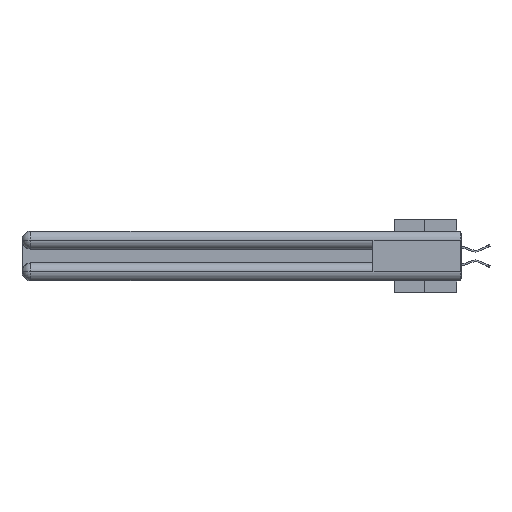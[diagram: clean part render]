
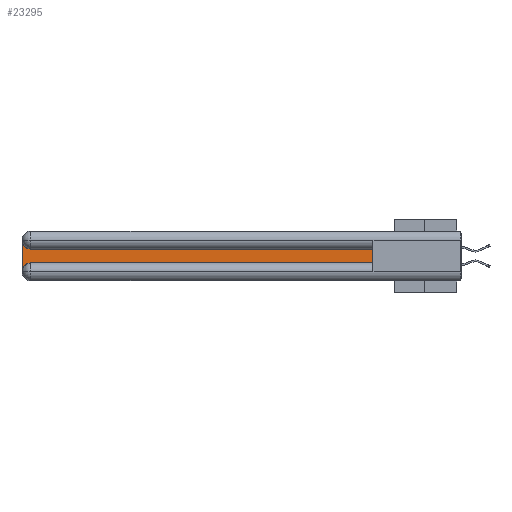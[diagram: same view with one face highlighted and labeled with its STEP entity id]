
A CAD part, left-side view. The second image highlights one B-rep face of the part: STEP entity #23295.
In plain terms, the highlighted planar face has unit normal (-1, 0, 0).
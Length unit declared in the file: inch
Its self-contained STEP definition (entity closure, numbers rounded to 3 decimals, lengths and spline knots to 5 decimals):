
#2069 = ORIENTED_EDGE ( 'NONE', *, *, #46272, .T. ) ;
#2218 = CIRCLE ( 'NONE', #29656, 0.06 ) ;
#2389 = CARTESIAN_POINT ( 'NONE',  ( 0.075, 0.6, -0.1225 ) ) ;
#2857 = LINE ( 'NONE', #18264, #46001 ) ;
#3168 = ORIENTED_EDGE ( 'NONE', *, *, #39112, .T. ) ;
#5815 = DIRECTION ( 'NONE',  ( 0., 1., 0. ) ) ;
#6115 = VERTEX_POINT ( 'NONE', #44631 ) ;
#7682 = DIRECTION ( 'NONE',  ( 1., 0., 0. ) ) ;
#7932 = CARTESIAN_POINT ( 'NONE',  ( 0.075, 2.94, -0.0625 ) ) ;
#8940 = VERTEX_POINT ( 'NONE', #38686 ) ;
#10243 = CARTESIAN_POINT ( 'NONE',  ( 0.075, 3., -0.2175 ) ) ;
#10977 = CARTESIAN_POINT ( 'NONE',  ( 0.075, 3., -0.2775 ) ) ;
#11154 = VERTEX_POINT ( 'NONE', #20081 ) ;
#11517 = DIRECTION ( 'NONE',  ( 0., 0., -1. ) ) ;
#12736 = FACE_OUTER_BOUND ( 'NONE', #31958, .T. ) ;
#13480 = ORIENTED_EDGE ( 'NONE', *, *, #30019, .T. ) ;
#13615 = AXIS2_PLACEMENT_3D ( 'NONE', #16270, #34154, #30084 ) ;
#15147 = DIRECTION ( 'NONE',  ( 0., 0., -1. ) ) ;
#15206 = ORIENTED_EDGE ( 'NONE', *, *, #25085, .T. ) ;
#16270 = CARTESIAN_POINT ( 'NONE',  ( 0.075, 3., -0.1225 ) ) ;
#16906 = VERTEX_POINT ( 'NONE', #38642 ) ;
#18264 = CARTESIAN_POINT ( 'NONE',  ( 0.075, 0.6, -0.2175 ) ) ;
#18644 = VECTOR ( 'NONE', #5815, 39.37008 ) ;
#20060 = EDGE_CURVE ( 'NONE', #16906, #21337, #37112, .T. ) ;
#20081 = CARTESIAN_POINT ( 'NONE',  ( 0.075, 0.6, -0.1225 ) ) ;
#20177 = CARTESIAN_POINT ( 'NONE',  ( 0.075, 3., -0.0625 ) ) ;
#21267 = DIRECTION ( 'NONE',  ( 0., 0., 1. ) ) ;
#21337 = VERTEX_POINT ( 'NONE', #20177 ) ;
#23295 = ADVANCED_FACE ( 'NONE', ( #12736 ), #37901, .F. ) ;
#24305 = VECTOR ( 'NONE', #21267, 39.37008 ) ;
#25085 = EDGE_CURVE ( 'NONE', #8940, #11154, #32155, .T. ) ;
#25297 = EDGE_CURVE ( 'NONE', #11154, #16906, #36591, .T. ) ;
#26817 = ORIENTED_EDGE ( 'NONE', *, *, #25297, .T. ) ;
#28229 = DIRECTION ( 'NONE',  ( 0., 0., -1. ) ) ;
#29656 = AXIS2_PLACEMENT_3D ( 'NONE', #32863, #7682, #15147 ) ;
#30019 = EDGE_CURVE ( 'NONE', #21337, #34014, #42413, .T. ) ;
#30084 = DIRECTION ( 'NONE',  ( 0., 0., -1. ) ) ;
#31958 = EDGE_LOOP ( 'NONE', ( #26817, #36513, #13480, #2069, #3168, #15206 ) ) ;
#32155 = LINE ( 'NONE', #43114, #24305 ) ;
#32863 = CARTESIAN_POINT ( 'NONE',  ( 0.075, 2.94, -0.2775 ) ) ;
#34014 = VERTEX_POINT ( 'NONE', #10977 ) ;
#34154 = DIRECTION ( 'NONE',  ( 1., 0., 0. ) ) ;
#36513 = ORIENTED_EDGE ( 'NONE', *, *, #20060, .T. ) ;
#36591 = LINE ( 'NONE', #2389, #18644 ) ;
#36714 = DIRECTION ( 'NONE',  ( 1., 0., 0. ) ) ;
#37112 = CIRCLE ( 'NONE', #39995, 0.06 ) ;
#37901 = PLANE ( 'NONE',  #13615 ) ;
#38642 = CARTESIAN_POINT ( 'NONE',  ( 0.075, 2.94, -0.1225 ) ) ;
#38686 = CARTESIAN_POINT ( 'NONE',  ( 0.075, 0.6, -0.2175 ) ) ;
#39112 = EDGE_CURVE ( 'NONE', #6115, #8940, #2857, .T. ) ;
#39148 = DIRECTION ( 'NONE',  ( 0., -1., 0. ) ) ;
#39995 = AXIS2_PLACEMENT_3D ( 'NONE', #7932, #36714, #11517 ) ;
#40729 = VECTOR ( 'NONE', #28229, 39.37008 ) ;
#42413 = LINE ( 'NONE', #10243, #40729 ) ;
#43114 = CARTESIAN_POINT ( 'NONE',  ( 0.075, 0.6, -0.2175 ) ) ;
#44631 = CARTESIAN_POINT ( 'NONE',  ( 0.075, 2.94, -0.2175 ) ) ;
#46001 = VECTOR ( 'NONE', #39148, 39.37008 ) ;
#46272 = EDGE_CURVE ( 'NONE', #34014, #6115, #2218, .T. ) ;
